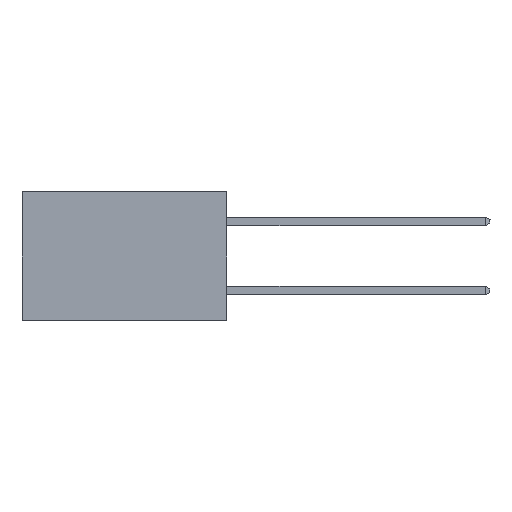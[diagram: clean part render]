
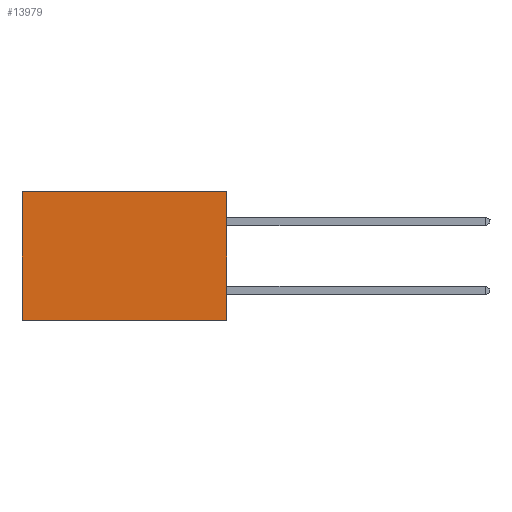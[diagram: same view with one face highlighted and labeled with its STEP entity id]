
A CAD part, left-side view. The second image highlights one B-rep face of the part: STEP entity #13979.
In plain terms, the highlighted planar face has unit normal (-1, 0, 0).
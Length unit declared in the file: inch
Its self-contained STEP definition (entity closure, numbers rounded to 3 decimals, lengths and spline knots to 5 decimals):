
#568 = VECTOR ( 'NONE', #4997, 39.37008 ) ;
#622 = DIRECTION ( 'NONE',  ( 0., 1., 0. ) ) ;
#654 = VERTEX_POINT ( 'NONE', #2284 ) ;
#2284 = CARTESIAN_POINT ( 'NONE',  ( 0.277, 0., -0.37 ) ) ;
#3563 = CARTESIAN_POINT ( 'NONE',  ( 0.277, 0., -0.37 ) ) ;
#3892 = CARTESIAN_POINT ( 'NONE',  ( 0.277, 0., -0.37 ) ) ;
#4013 = AXIS2_PLACEMENT_3D ( 'NONE', #3563, #7857, #22728 ) ;
#4252 = VERTEX_POINT ( 'NONE', #20457 ) ;
#4997 = DIRECTION ( 'NONE',  ( 0., 0., -1. ) ) ;
#5412 = VECTOR ( 'NONE', #6045, 39.37008 ) ;
#5711 = VECTOR ( 'NONE', #22737, 39.37008 ) ;
#5724 = PLANE ( 'NONE',  #4013 ) ;
#6045 = DIRECTION ( 'NONE',  ( 0., 0., -1. ) ) ;
#6293 = LINE ( 'NONE', #26002, #568 ) ;
#6481 = EDGE_LOOP ( 'NONE', ( #15283, #21881, #12344, #10773 ) ) ;
#7857 = DIRECTION ( 'NONE',  ( 1., 0., 0. ) ) ;
#9507 = EDGE_CURVE ( 'NONE', #23437, #4252, #12773, .T. ) ;
#10773 = ORIENTED_EDGE ( 'NONE', *, *, #9507, .T. ) ;
#11390 = LINE ( 'NONE', #18517, #5711 ) ;
#12105 = VECTOR ( 'NONE', #622, 39.37008 ) ;
#12344 = ORIENTED_EDGE ( 'NONE', *, *, #26680, .F. ) ;
#12773 = LINE ( 'NONE', #23971, #12105 ) ;
#13751 = FACE_OUTER_BOUND ( 'NONE', #6481, .T. ) ;
#13979 = ADVANCED_FACE ( 'NONE', ( #13751 ), #5724, .F. ) ;
#14336 = EDGE_CURVE ( 'NONE', #654, #25170, #11390, .T. ) ;
#15283 = ORIENTED_EDGE ( 'NONE', *, *, #22515, .T. ) ;
#15436 = LINE ( 'NONE', #3892, #5412 ) ;
#18517 = CARTESIAN_POINT ( 'NONE',  ( 0.277, 0., -0.37 ) ) ;
#20457 = CARTESIAN_POINT ( 'NONE',  ( 0.277, 0.59, 0. ) ) ;
#21881 = ORIENTED_EDGE ( 'NONE', *, *, #14336, .F. ) ;
#22515 = EDGE_CURVE ( 'NONE', #4252, #25170, #6293, .T. ) ;
#22728 = DIRECTION ( 'NONE',  ( 0., 0., -1. ) ) ;
#22737 = DIRECTION ( 'NONE',  ( 0., 1., 0. ) ) ;
#22798 = CARTESIAN_POINT ( 'NONE',  ( 0.277, 0., 0. ) ) ;
#23437 = VERTEX_POINT ( 'NONE', #22798 ) ;
#23971 = CARTESIAN_POINT ( 'NONE',  ( 0.277, 0., 0. ) ) ;
#25170 = VERTEX_POINT ( 'NONE', #26731 ) ;
#26002 = CARTESIAN_POINT ( 'NONE',  ( 0.277, 0.59, -0.37 ) ) ;
#26680 = EDGE_CURVE ( 'NONE', #23437, #654, #15436, .T. ) ;
#26731 = CARTESIAN_POINT ( 'NONE',  ( 0.277, 0.59, -0.37 ) ) ;
